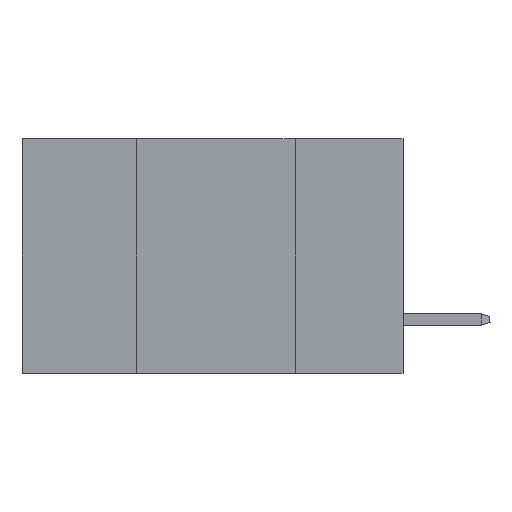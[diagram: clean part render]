
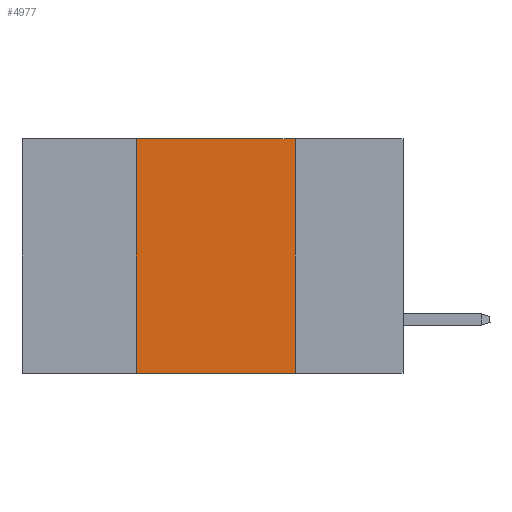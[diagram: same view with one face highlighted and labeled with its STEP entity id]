
A CAD part, left-side view. The second image highlights one B-rep face of the part: STEP entity #4977.
In plain terms, the highlighted planar face has unit normal (-1, 0, 0).
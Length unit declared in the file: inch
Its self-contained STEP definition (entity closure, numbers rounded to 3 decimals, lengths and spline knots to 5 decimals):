
#188 = DIRECTION ( 'NONE',  ( 1., 0., 0. ) ) ;
#299 = VECTOR ( 'NONE', #17983, 39.37008 ) ;
#1523 = ORIENTED_EDGE ( 'NONE', *, *, #13497, .T. ) ;
#1846 = ORIENTED_EDGE ( 'NONE', *, *, #13957, .F. ) ;
#2016 = VERTEX_POINT ( 'NONE', #11880 ) ;
#2557 = CARTESIAN_POINT ( 'NONE',  ( 0., 0.42, 0. ) ) ;
#3491 = DIRECTION ( 'NONE',  ( 0., 0., 1. ) ) ;
#4516 = FACE_OUTER_BOUND ( 'NONE', #17271, .T. ) ;
#4610 = CARTESIAN_POINT ( 'NONE',  ( 0., 0.17, 0. ) ) ;
#4977 = ADVANCED_FACE ( 'NONE', ( #4516 ), #10525, .F. ) ;
#5195 = DIRECTION ( 'NONE',  ( 0., -1., 0. ) ) ;
#6353 = VECTOR ( 'NONE', #5195, 39.37008 ) ;
#7899 = CARTESIAN_POINT ( 'NONE',  ( 0., 0.6, -0.37 ) ) ;
#8176 = VERTEX_POINT ( 'NONE', #4610 ) ;
#8740 = ORIENTED_EDGE ( 'NONE', *, *, #10916, .F. ) ;
#8970 = LINE ( 'NONE', #9072, #299 ) ;
#8983 = CARTESIAN_POINT ( 'NONE',  ( 0., 0.42, -0.37 ) ) ;
#9072 = CARTESIAN_POINT ( 'NONE',  ( 0., 0.17, 0. ) ) ;
#9271 = VERTEX_POINT ( 'NONE', #2557 ) ;
#9493 = VECTOR ( 'NONE', #18091, 39.37008 ) ;
#10525 = PLANE ( 'NONE',  #12510 ) ;
#10916 = EDGE_CURVE ( 'NONE', #8176, #2016, #8970, .T. ) ;
#11880 = CARTESIAN_POINT ( 'NONE',  ( 0., 0.17, -0.37 ) ) ;
#12510 = AXIS2_PLACEMENT_3D ( 'NONE', #18060, #188, #18169 ) ;
#12758 = CARTESIAN_POINT ( 'NONE',  ( 0., 0.6, 0. ) ) ;
#13497 = EDGE_CURVE ( 'NONE', #14823, #2016, #17893, .T. ) ;
#13912 = CARTESIAN_POINT ( 'NONE',  ( 0., 0.42, 0. ) ) ;
#13957 = EDGE_CURVE ( 'NONE', #9271, #8176, #15517, .T. ) ;
#14823 = VERTEX_POINT ( 'NONE', #8983 ) ;
#15194 = LINE ( 'NONE', #13912, #18626 ) ;
#15517 = LINE ( 'NONE', #12758, #6353 ) ;
#15641 = EDGE_CURVE ( 'NONE', #14823, #9271, #15194, .T. ) ;
#17271 = EDGE_LOOP ( 'NONE', ( #8740, #1846, #18302, #1523 ) ) ;
#17893 = LINE ( 'NONE', #7899, #9493 ) ;
#17983 = DIRECTION ( 'NONE',  ( 0., 0., -1. ) ) ;
#18060 = CARTESIAN_POINT ( 'NONE',  ( 0., 0.6, 0. ) ) ;
#18091 = DIRECTION ( 'NONE',  ( 0., -1., 0. ) ) ;
#18169 = DIRECTION ( 'NONE',  ( 0., 0., -1. ) ) ;
#18302 = ORIENTED_EDGE ( 'NONE', *, *, #15641, .F. ) ;
#18626 = VECTOR ( 'NONE', #3491, 39.37008 ) ;
